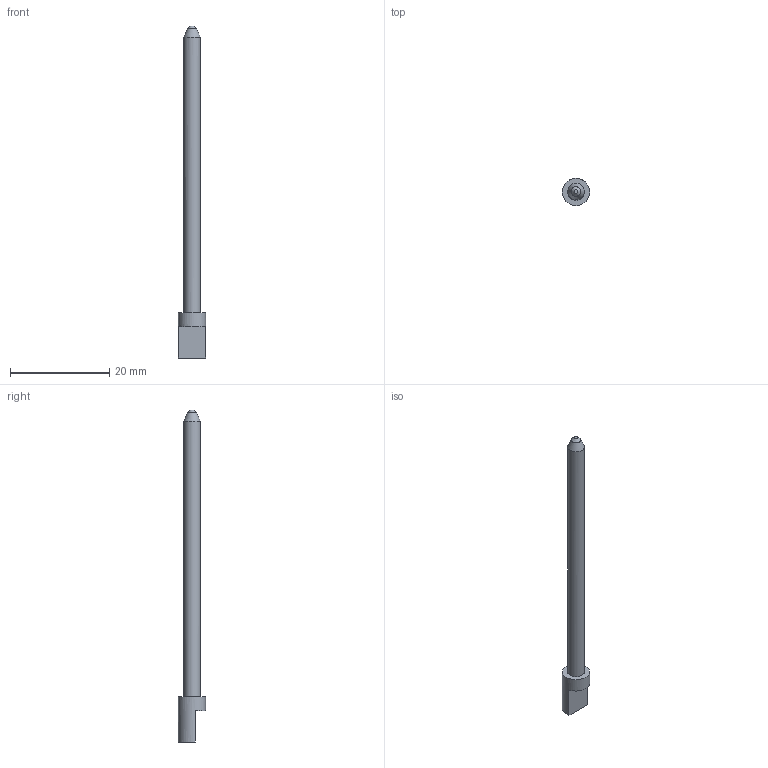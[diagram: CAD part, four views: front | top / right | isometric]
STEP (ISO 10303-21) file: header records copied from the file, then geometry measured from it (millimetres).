
FILE_DESCRIPTION(('FreeCAD Model'),'2;1');
FILE_NAME('simulated firing pin.step' ,'2015-07-10T13:29:33',('Author'),(''), 'Open CASCADE STEP processor 6.8','FreeCAD','Unknown');
FILE_SCHEMA(('AUTOMOTIVE_DESIGN_CC2 { 1 2 10303 214 -1 1 5 4 }'));
Length unit declared in the file: millimetre
Products named in the file (1): Pocket
Bounding box: 5.5 x 5.5 x 66.9 mm (x, y, z)
Volume: 663.5 mm3; surface area: 786.9 mm2
Topology: 1 solids, 1 shells, 9 faces, 16 edges, 10 vertices
Faces by surface type: plane 5, cylinder 2, bspline 1, cone 1
Full cylindrical faces by diameter (mm): 3.35 x1, 5.5 x1
Entity records: 565 total; most frequent: CARTESIAN_POINT 228, DIRECTION 54, ORIENTED_EDGE 32, PCURVE 32, DEFINITIONAL_REPRESENTATION 32, LINE 23, VECTOR 23, EDGE_CURVE 16
